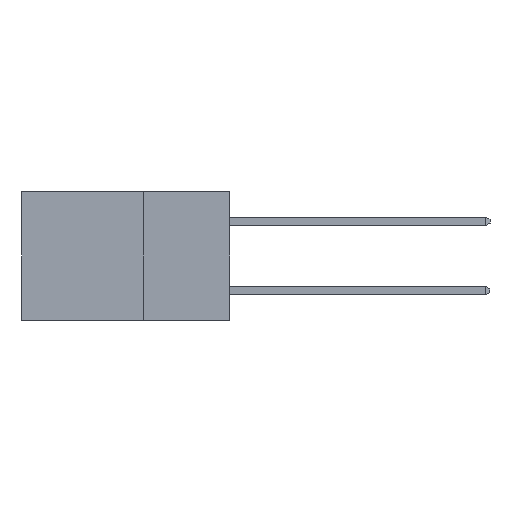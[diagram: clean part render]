
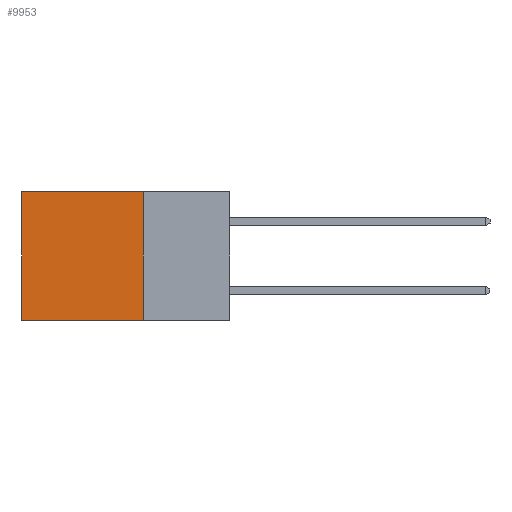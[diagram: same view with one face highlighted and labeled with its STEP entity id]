
A CAD part, left-side view. The second image highlights one B-rep face of the part: STEP entity #9953.
In plain terms, the highlighted planar face has unit normal (-1, 0, 0).
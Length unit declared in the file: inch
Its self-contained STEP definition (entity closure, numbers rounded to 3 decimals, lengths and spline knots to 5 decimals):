
#61 = LINE ( 'NONE', #9815, #14823 ) ;
#407 = DIRECTION ( 'NONE',  ( 1., 0., 0. ) ) ;
#468 = VERTEX_POINT ( 'NONE', #8554 ) ;
#765 = DIRECTION ( 'NONE',  ( 0., 1., 0. ) ) ;
#902 = DIRECTION ( 'NONE',  ( 0., 0., -1. ) ) ;
#1036 = EDGE_CURVE ( 'NONE', #5952, #7918, #61, .T. ) ;
#1787 = VECTOR ( 'NONE', #9838, 39.37008 ) ;
#1957 = EDGE_LOOP ( 'NONE', ( #15510, #6637, #15251, #9653 ) ) ;
#2258 = EDGE_CURVE ( 'NONE', #5952, #9347, #13247, .T. ) ;
#4094 = CARTESIAN_POINT ( 'NONE',  ( 0.298, 0.6, 0. ) ) ;
#4323 = VECTOR ( 'NONE', #765, 39.37008 ) ;
#5952 = VERTEX_POINT ( 'NONE', #11006 ) ;
#6554 = CARTESIAN_POINT ( 'NONE',  ( 0.298, 0.25, -0.37 ) ) ;
#6637 = ORIENTED_EDGE ( 'NONE', *, *, #6846, .F. ) ;
#6846 = EDGE_CURVE ( 'NONE', #7918, #468, #12429, .T. ) ;
#7918 = VERTEX_POINT ( 'NONE', #12102 ) ;
#8249 = EDGE_CURVE ( 'NONE', #9347, #468, #14349, .T. ) ;
#8554 = CARTESIAN_POINT ( 'NONE',  ( 0.298, 0.6, -0.37 ) ) ;
#9016 = CARTESIAN_POINT ( 'NONE',  ( 0.298, 0.25, 0. ) ) ;
#9347 = VERTEX_POINT ( 'NONE', #16310 ) ;
#9653 = ORIENTED_EDGE ( 'NONE', *, *, #2258, .T. ) ;
#9815 = CARTESIAN_POINT ( 'NONE',  ( 0.298, 0.25, 0. ) ) ;
#9838 = DIRECTION ( 'NONE',  ( 0., 1., 0. ) ) ;
#9953 = ADVANCED_FACE ( 'NONE', ( #15161 ), #16108, .F. ) ;
#9994 = CARTESIAN_POINT ( 'NONE',  ( 0.298, 0.25, 0. ) ) ;
#10481 = DIRECTION ( 'NONE',  ( 0., 0., -1. ) ) ;
#11006 = CARTESIAN_POINT ( 'NONE',  ( 0.298, 0.25, 0. ) ) ;
#12102 = CARTESIAN_POINT ( 'NONE',  ( 0.298, 0.25, -0.37 ) ) ;
#12429 = LINE ( 'NONE', #6554, #4323 ) ;
#13247 = LINE ( 'NONE', #9994, #1787 ) ;
#14349 = LINE ( 'NONE', #4094, #18064 ) ;
#14823 = VECTOR ( 'NONE', #902, 39.37008 ) ;
#15161 = FACE_OUTER_BOUND ( 'NONE', #1957, .T. ) ;
#15251 = ORIENTED_EDGE ( 'NONE', *, *, #1036, .F. ) ;
#15510 = ORIENTED_EDGE ( 'NONE', *, *, #8249, .T. ) ;
#15541 = DIRECTION ( 'NONE',  ( 0., 0., -1. ) ) ;
#16108 = PLANE ( 'NONE',  #17986 ) ;
#16310 = CARTESIAN_POINT ( 'NONE',  ( 0.298, 0.6, 0. ) ) ;
#17986 = AXIS2_PLACEMENT_3D ( 'NONE', #9016, #407, #10481 ) ;
#18064 = VECTOR ( 'NONE', #15541, 39.37008 ) ;
